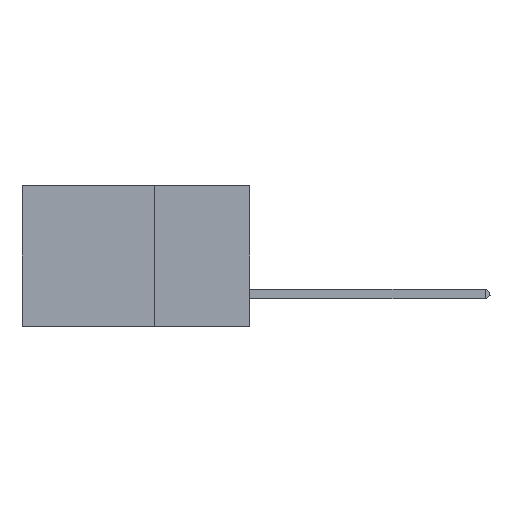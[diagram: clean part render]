
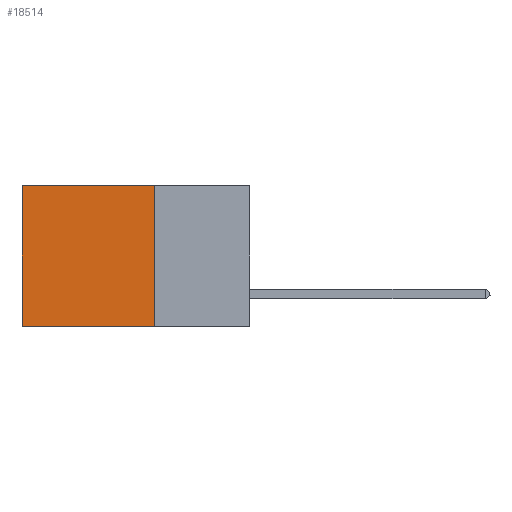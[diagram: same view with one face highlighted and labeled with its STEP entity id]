
A CAD part, left-side view. The second image highlights one B-rep face of the part: STEP entity #18514.
In plain terms, the highlighted planar face has unit normal (-1, 0, 0).
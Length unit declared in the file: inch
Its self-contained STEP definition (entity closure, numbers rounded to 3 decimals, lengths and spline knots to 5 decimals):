
#787 = VECTOR ( 'NONE', #15168, 39.37008 ) ;
#1442 = AXIS2_PLACEMENT_3D ( 'NONE', #6244, #30443, #40147 ) ;
#1514 = EDGE_LOOP ( 'NONE', ( #28840, #33167, #43865, #7290 ) ) ;
#2063 = FACE_OUTER_BOUND ( 'NONE', #1514, .T. ) ;
#2985 = LINE ( 'NONE', #8106, #787 ) ;
#3207 = CARTESIAN_POINT ( 'NONE',  ( 0.2875, 0.25, -0.37 ) ) ;
#4599 = CARTESIAN_POINT ( 'NONE',  ( 0.2875, 0.25, 0. ) ) ;
#6244 = CARTESIAN_POINT ( 'NONE',  ( 0.2875, 0.25, 0. ) ) ;
#7290 = ORIENTED_EDGE ( 'NONE', *, *, #15109, .T. ) ;
#7304 = VERTEX_POINT ( 'NONE', #4599 ) ;
#7897 = VECTOR ( 'NONE', #11847, 39.37008 ) ;
#8106 = CARTESIAN_POINT ( 'NONE',  ( 0.2875, 0.25, -0.37 ) ) ;
#9942 = CARTESIAN_POINT ( 'NONE',  ( 0.2875, 0.6, -0.37 ) ) ;
#10172 = VECTOR ( 'NONE', #29213, 39.37008 ) ;
#10583 = VECTOR ( 'NONE', #39809, 39.37008 ) ;
#11847 = DIRECTION ( 'NONE',  ( 0., 0., -1. ) ) ;
#13738 = EDGE_CURVE ( 'NONE', #7304, #17432, #37193, .T. ) ;
#15109 = EDGE_CURVE ( 'NONE', #7304, #41641, #15455, .T. ) ;
#15168 = DIRECTION ( 'NONE',  ( 0., 1., 0. ) ) ;
#15455 = LINE ( 'NONE', #22467, #10583 ) ;
#17432 = VERTEX_POINT ( 'NONE', #3207 ) ;
#18514 = ADVANCED_FACE ( 'NONE', ( #2063 ), #26502, .F. ) ;
#22151 = CARTESIAN_POINT ( 'NONE',  ( 0.2875, 0.25, 0. ) ) ;
#22467 = CARTESIAN_POINT ( 'NONE',  ( 0.2875, 0.25, 0. ) ) ;
#22490 = LINE ( 'NONE', #32538, #7897 ) ;
#26502 = PLANE ( 'NONE',  #1442 ) ;
#28840 = ORIENTED_EDGE ( 'NONE', *, *, #32737, .T. ) ;
#29213 = DIRECTION ( 'NONE',  ( 0., 0., -1. ) ) ;
#30443 = DIRECTION ( 'NONE',  ( 1., 0., 0. ) ) ;
#32538 = CARTESIAN_POINT ( 'NONE',  ( 0.2875, 0.6, 0. ) ) ;
#32737 = EDGE_CURVE ( 'NONE', #41641, #42386, #22490, .T. ) ;
#33167 = ORIENTED_EDGE ( 'NONE', *, *, #38294, .F. ) ;
#35681 = CARTESIAN_POINT ( 'NONE',  ( 0.2875, 0.6, 0. ) ) ;
#37193 = LINE ( 'NONE', #22151, #10172 ) ;
#38294 = EDGE_CURVE ( 'NONE', #17432, #42386, #2985, .T. ) ;
#39809 = DIRECTION ( 'NONE',  ( 0., 1., 0. ) ) ;
#40147 = DIRECTION ( 'NONE',  ( 0., 0., -1. ) ) ;
#41641 = VERTEX_POINT ( 'NONE', #35681 ) ;
#42386 = VERTEX_POINT ( 'NONE', #9942 ) ;
#43865 = ORIENTED_EDGE ( 'NONE', *, *, #13738, .F. ) ;
